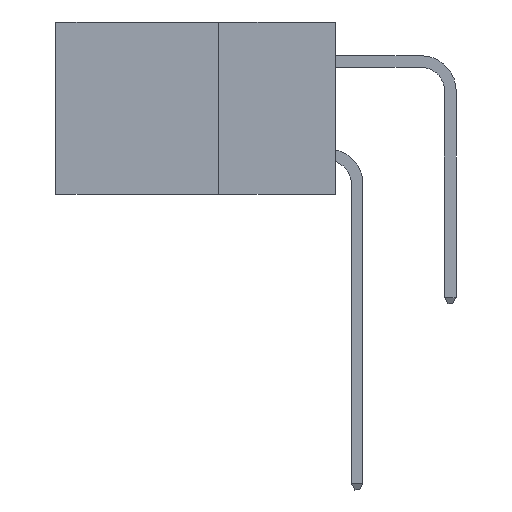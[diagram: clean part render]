
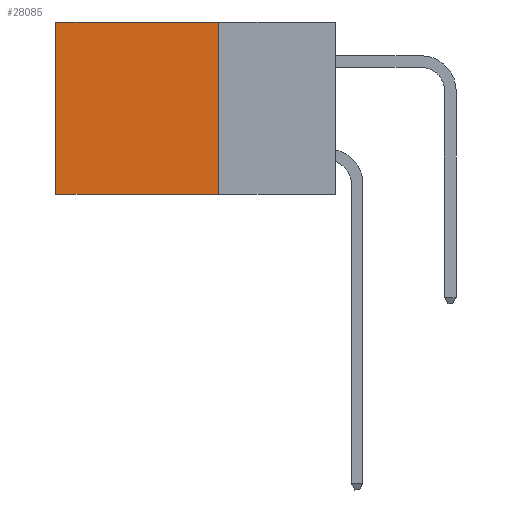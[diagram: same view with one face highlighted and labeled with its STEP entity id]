
A CAD part, left-side view. The second image highlights one B-rep face of the part: STEP entity #28085.
In plain terms, the highlighted planar face has unit normal (-1, 0, 0).
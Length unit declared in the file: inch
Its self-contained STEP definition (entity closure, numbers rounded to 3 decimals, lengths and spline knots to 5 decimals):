
#4037 = FACE_OUTER_BOUND ( 'NONE', #27317, .T. ) ;
#6368 = CARTESIAN_POINT ( 'NONE',  ( 0.2875, 0.25, -0.37 ) ) ;
#7928 = LINE ( 'NONE', #26261, #24806 ) ;
#8156 = CARTESIAN_POINT ( 'NONE',  ( 0.2875, 0.25, -0.37 ) ) ;
#8401 = CARTESIAN_POINT ( 'NONE',  ( 0.2875, 0.6, 0. ) ) ;
#9105 = EDGE_CURVE ( 'NONE', #40772, #32330, #7928, .T. ) ;
#9135 = ORIENTED_EDGE ( 'NONE', *, *, #11487, .F. ) ;
#11487 = EDGE_CURVE ( 'NONE', #40772, #27048, #38127, .T. ) ;
#11957 = VECTOR ( 'NONE', #29857, 39.37008 ) ;
#12439 = DIRECTION ( 'NONE',  ( 0., 1., 0. ) ) ;
#13029 = EDGE_CURVE ( 'NONE', #32330, #14386, #35343, .T. ) ;
#13405 = CARTESIAN_POINT ( 'NONE',  ( 0.2875, 0.25, 0. ) ) ;
#13695 = VECTOR ( 'NONE', #28439, 39.37008 ) ;
#14386 = VERTEX_POINT ( 'NONE', #42916 ) ;
#15203 = CARTESIAN_POINT ( 'NONE',  ( 0.2875, 0.25, 0. ) ) ;
#19949 = ORIENTED_EDGE ( 'NONE', *, *, #33176, .F. ) ;
#24218 = AXIS2_PLACEMENT_3D ( 'NONE', #13405, #31034, #37692 ) ;
#24806 = VECTOR ( 'NONE', #12439, 39.37008 ) ;
#26261 = CARTESIAN_POINT ( 'NONE',  ( 0.2875, 0.25, 0. ) ) ;
#27048 = VERTEX_POINT ( 'NONE', #8156 ) ;
#27317 = EDGE_LOOP ( 'NONE', ( #30092, #19949, #9135, #41899 ) ) ;
#28085 = ADVANCED_FACE ( 'NONE', ( #4037 ), #34238, .F. ) ;
#28439 = DIRECTION ( 'NONE',  ( 0., 0., -1. ) ) ;
#29857 = DIRECTION ( 'NONE',  ( 0., 0., -1. ) ) ;
#30092 = ORIENTED_EDGE ( 'NONE', *, *, #13029, .T. ) ;
#30894 = CARTESIAN_POINT ( 'NONE',  ( 0.2875, 0.25, 0. ) ) ;
#31034 = DIRECTION ( 'NONE',  ( 1., 0., 0. ) ) ;
#32330 = VERTEX_POINT ( 'NONE', #8401 ) ;
#33176 = EDGE_CURVE ( 'NONE', #27048, #14386, #34862, .T. ) ;
#34238 = PLANE ( 'NONE',  #24218 ) ;
#34862 = LINE ( 'NONE', #6368, #38578 ) ;
#35343 = LINE ( 'NONE', #43602, #11957 ) ;
#37692 = DIRECTION ( 'NONE',  ( 0., 0., -1. ) ) ;
#38127 = LINE ( 'NONE', #30894, #13695 ) ;
#38578 = VECTOR ( 'NONE', #40938, 39.37008 ) ;
#40772 = VERTEX_POINT ( 'NONE', #15203 ) ;
#40938 = DIRECTION ( 'NONE',  ( 0., 1., 0. ) ) ;
#41899 = ORIENTED_EDGE ( 'NONE', *, *, #9105, .T. ) ;
#42916 = CARTESIAN_POINT ( 'NONE',  ( 0.2875, 0.6, -0.37 ) ) ;
#43602 = CARTESIAN_POINT ( 'NONE',  ( 0.2875, 0.6, 0. ) ) ;
